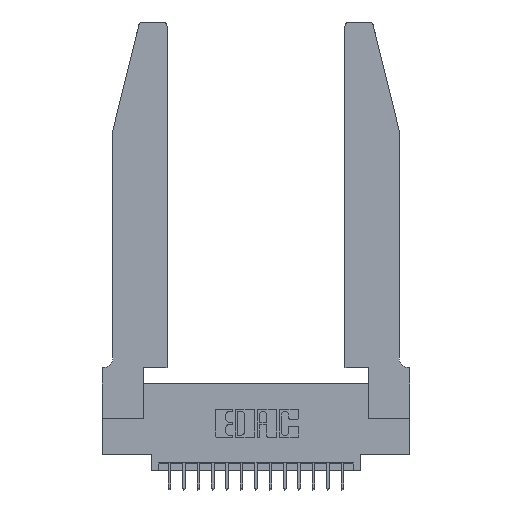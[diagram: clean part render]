
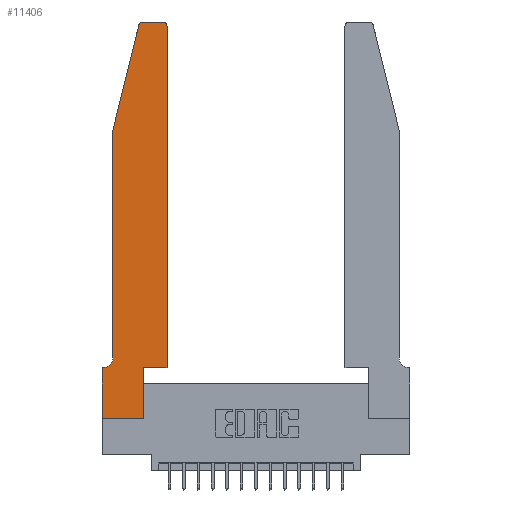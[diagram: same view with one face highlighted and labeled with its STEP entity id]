
A CAD part, top view. The second image highlights one B-rep face of the part: STEP entity #11406.
In plain terms, the highlighted planar face has unit normal (0, 0, 1).
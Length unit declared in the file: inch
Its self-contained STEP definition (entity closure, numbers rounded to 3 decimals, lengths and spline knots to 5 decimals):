
#3 = CARTESIAN_POINT ( 'NONE',  ( 0.0055, 0.35, 0.37 ) ) ;
#127 = ORIENTED_EDGE ( 'NONE', *, *, #9507, .T. ) ;
#208 = CARTESIAN_POINT ( 'NONE',  ( 0., 0., 0.37 ) ) ;
#465 = CARTESIAN_POINT ( 'NONE',  ( 0.0755, 0.35, 0.37 ) ) ;
#482 = EDGE_CURVE ( 'NONE', #3838, #14327, #3735, .T. ) ;
#611 = CARTESIAN_POINT ( 'NONE',  ( 0.0755, 0.42, 0.37 ) ) ;
#1259 = ORIENTED_EDGE ( 'NONE', *, *, #2839, .T. ) ;
#1329 = LINE ( 'NONE', #8450, #11074 ) ;
#1384 = EDGE_CURVE ( 'NONE', #3852, #3607, #1329, .T. ) ;
#1509 = CARTESIAN_POINT ( 'NONE',  ( 0.4205, 2.75, 0.37 ) ) ;
#1590 = ORIENTED_EDGE ( 'NONE', *, *, #6439, .T. ) ;
#1628 = EDGE_CURVE ( 'NONE', #7120, #14860, #17567, .T. ) ;
#1681 = CARTESIAN_POINT ( 'NONE',  ( 0.0755, 2., 0.37 ) ) ;
#1752 = DIRECTION ( 'NONE',  ( 1., 0., 0. ) ) ;
#2008 = DIRECTION ( 'NONE',  ( -1., 0., 0. ) ) ;
#2149 = CARTESIAN_POINT ( 'NONE',  ( 0.2865, 0., 0.37 ) ) ;
#2644 = VECTOR ( 'NONE', #2008, 39.37008 ) ;
#2839 = EDGE_CURVE ( 'NONE', #5332, #3852, #4193, .T. ) ;
#3271 = VECTOR ( 'NONE', #11592, 39.37008 ) ;
#3315 = CARTESIAN_POINT ( 'NONE',  ( 0.0055, 0.42, 0.37 ) ) ;
#3607 = VERTEX_POINT ( 'NONE', #17251 ) ;
#3735 = CIRCLE ( 'NONE', #6212, 0.07 ) ;
#3838 = VERTEX_POINT ( 'NONE', #611 ) ;
#3852 = VERTEX_POINT ( 'NONE', #2149 ) ;
#4193 = LINE ( 'NONE', #10015, #8026 ) ;
#4201 = ORIENTED_EDGE ( 'NONE', *, *, #11989, .T. ) ;
#4622 = LINE ( 'NONE', #16382, #15721 ) ;
#4639 = CARTESIAN_POINT ( 'NONE',  ( 0.4505, 0.35, 0.37 ) ) ;
#4978 = DIRECTION ( 'NONE',  ( 0., 0., 1. ) ) ;
#5332 = VERTEX_POINT ( 'NONE', #208 ) ;
#5384 = DIRECTION ( 'NONE',  ( 0., 0., 1. ) ) ;
#5412 = CARTESIAN_POINT ( 'NONE',  ( 0.0755, 2., 0.37 ) ) ;
#5632 = EDGE_CURVE ( 'NONE', #14860, #14706, #18790, .T. ) ;
#5749 = LINE ( 'NONE', #13250, #3271 ) ;
#5822 = CARTESIAN_POINT ( 'NONE',  ( 0.4505, 0.35, 0.37 ) ) ;
#5828 = FACE_OUTER_BOUND ( 'NONE', #7765, .T. ) ;
#5839 = DIRECTION ( 'NONE',  ( 1., 0., 0. ) ) ;
#5938 = VECTOR ( 'NONE', #1752, 39.37008 ) ;
#6099 = PLANE ( 'NONE',  #6602 ) ;
#6212 = AXIS2_PLACEMENT_3D ( 'NONE', #3315, #14580, #19046 ) ;
#6439 = EDGE_CURVE ( 'NONE', #12591, #7120, #4622, .T. ) ;
#6545 = LINE ( 'NONE', #465, #2644 ) ;
#6602 = AXIS2_PLACEMENT_3D ( 'NONE', #10307, #12055, #17950 ) ;
#6722 = ORIENTED_EDGE ( 'NONE', *, *, #1384, .T. ) ;
#7020 = VERTEX_POINT ( 'NONE', #13357 ) ;
#7120 = VERTEX_POINT ( 'NONE', #14105 ) ;
#7496 = CARTESIAN_POINT ( 'NONE',  ( 0., 0.35, 0.37 ) ) ;
#7758 = DIRECTION ( 'NONE',  ( 0., -1., 0. ) ) ;
#7765 = EDGE_LOOP ( 'NONE', ( #8721, #8443, #4201, #15622, #18114, #16048, #13552, #1259, #6722, #127, #1590, #17038 ) ) ;
#7859 = DIRECTION ( 'NONE',  ( 1., 0., 0. ) ) ;
#8026 = VECTOR ( 'NONE', #5839, 39.37008 ) ;
#8443 = ORIENTED_EDGE ( 'NONE', *, *, #17743, .T. ) ;
#8450 = CARTESIAN_POINT ( 'NONE',  ( 0.2865, 0.35, 0.37 ) ) ;
#8665 = VECTOR ( 'NONE', #7758, 39.37008 ) ;
#8721 = ORIENTED_EDGE ( 'NONE', *, *, #5632, .T. ) ;
#8741 = EDGE_CURVE ( 'NONE', #12455, #3838, #16426, .T. ) ;
#9507 = EDGE_CURVE ( 'NONE', #3607, #12591, #16200, .T. ) ;
#10015 = CARTESIAN_POINT ( 'NONE',  ( 0., 0., 0.37 ) ) ;
#10307 = CARTESIAN_POINT ( 'NONE',  ( 0., 0.35, 0.37 ) ) ;
#11074 = VECTOR ( 'NONE', #17518, 39.37008 ) ;
#11406 = ADVANCED_FACE ( 'NONE', ( #5828 ), #6099, .T. ) ;
#11592 = DIRECTION ( 'NONE',  ( 0., -1., 0. ) ) ;
#11989 = EDGE_CURVE ( 'NONE', #7020, #12455, #18921, .T. ) ;
#12055 = DIRECTION ( 'NONE',  ( 0., 0., 1. ) ) ;
#12455 = VERTEX_POINT ( 'NONE', #1681 ) ;
#12591 = VERTEX_POINT ( 'NONE', #4639 ) ;
#13250 = CARTESIAN_POINT ( 'NONE',  ( 0., 0., 0.37 ) ) ;
#13357 = CARTESIAN_POINT ( 'NONE',  ( 0.25487, 2.72718, 0.37 ) ) ;
#13552 = ORIENTED_EDGE ( 'NONE', *, *, #15744, .T. ) ;
#13862 = AXIS2_PLACEMENT_3D ( 'NONE', #18591, #5384, #16748 ) ;
#14033 = VERTEX_POINT ( 'NONE', #7496 ) ;
#14105 = CARTESIAN_POINT ( 'NONE',  ( 0.4505, 2.72, 0.37 ) ) ;
#14327 = VERTEX_POINT ( 'NONE', #3 ) ;
#14525 = DIRECTION ( 'NONE',  ( -1., 0., 0. ) ) ;
#14580 = DIRECTION ( 'NONE',  ( 0., 0., -1. ) ) ;
#14608 = VECTOR ( 'NONE', #17440, 39.37008 ) ;
#14706 = VERTEX_POINT ( 'NONE', #14741 ) ;
#14741 = CARTESIAN_POINT ( 'NONE',  ( 0.284, 2.75, 0.37 ) ) ;
#14860 = VERTEX_POINT ( 'NONE', #1509 ) ;
#15622 = ORIENTED_EDGE ( 'NONE', *, *, #8741, .T. ) ;
#15721 = VECTOR ( 'NONE', #16468, 39.37008 ) ;
#15744 = EDGE_CURVE ( 'NONE', #14033, #5332, #5749, .T. ) ;
#15881 = CARTESIAN_POINT ( 'NONE',  ( 0.2605, 2.75, 0.37 ) ) ;
#16048 = ORIENTED_EDGE ( 'NONE', *, *, #16253, .T. ) ;
#16200 = LINE ( 'NONE', #5822, #5938 ) ;
#16241 = AXIS2_PLACEMENT_3D ( 'NONE', #16622, #4978, #7859 ) ;
#16253 = EDGE_CURVE ( 'NONE', #14327, #14033, #6545, .T. ) ;
#16382 = CARTESIAN_POINT ( 'NONE',  ( 0.4505, 0.35, 0.37 ) ) ;
#16426 = LINE ( 'NONE', #18079, #8665 ) ;
#16468 = DIRECTION ( 'NONE',  ( 0., 1., 0. ) ) ;
#16622 = CARTESIAN_POINT ( 'NONE',  ( 0.284, 2.72, 0.37 ) ) ;
#16748 = DIRECTION ( 'NONE',  ( 1., 0., 0. ) ) ;
#17038 = ORIENTED_EDGE ( 'NONE', *, *, #1628, .T. ) ;
#17251 = CARTESIAN_POINT ( 'NONE',  ( 0.2865, 0.35, 0.37 ) ) ;
#17440 = DIRECTION ( 'NONE',  ( -0.239, -0.971, 0. ) ) ;
#17518 = DIRECTION ( 'NONE',  ( 0., 1., 0. ) ) ;
#17567 = CIRCLE ( 'NONE', #13862, 0.03 ) ;
#17743 = EDGE_CURVE ( 'NONE', #14706, #7020, #18415, .T. ) ;
#17950 = DIRECTION ( 'NONE',  ( 1., 0., 0. ) ) ;
#18079 = CARTESIAN_POINT ( 'NONE',  ( 0.0755, 2., 0.37 ) ) ;
#18114 = ORIENTED_EDGE ( 'NONE', *, *, #482, .T. ) ;
#18415 = CIRCLE ( 'NONE', #16241, 0.03 ) ;
#18529 = VECTOR ( 'NONE', #14525, 39.37008 ) ;
#18591 = CARTESIAN_POINT ( 'NONE',  ( 0.4205, 2.72, 0.37 ) ) ;
#18790 = LINE ( 'NONE', #15881, #18529 ) ;
#18921 = LINE ( 'NONE', #5412, #14608 ) ;
#19046 = DIRECTION ( 'NONE',  ( -1., 0., 0. ) ) ;
